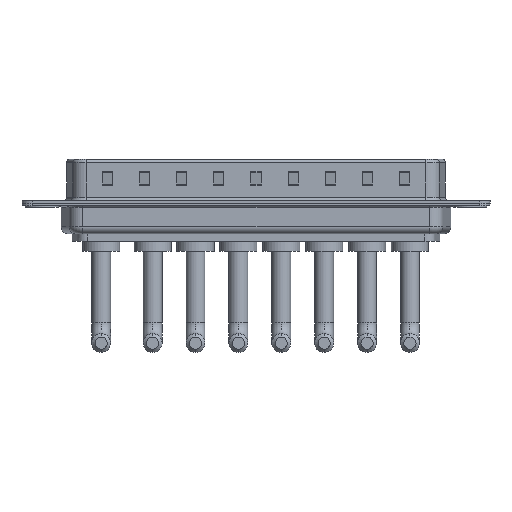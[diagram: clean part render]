
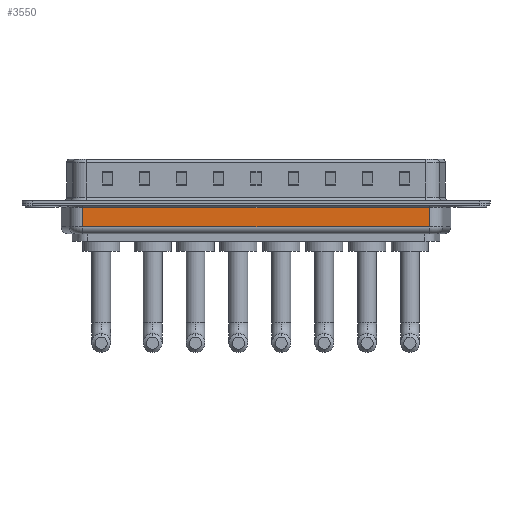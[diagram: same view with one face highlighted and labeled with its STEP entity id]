
A CAD part, front view. The second image highlights one B-rep face of the part: STEP entity #3550.
In plain terms, the highlighted planar face has unit normal (0, -1, 0).
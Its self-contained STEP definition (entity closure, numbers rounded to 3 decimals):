
#327 = ORIENTED_EDGE ( 'NONE', *, *, #14041, .T. ) ;
#1242 = CARTESIAN_POINT ( 'NONE',  ( 57.469, -5.35, -0.65 ) ) ;
#1476 = FACE_OUTER_BOUND ( 'NONE', #12144, .T. ) ;
#1701 = DIRECTION ( 'NONE',  ( 0., 0., 1. ) ) ;
#1750 = VERTEX_POINT ( 'NONE', #3593 ) ;
#2041 = EDGE_CURVE ( 'NONE', #8917, #1750, #11898, .T. ) ;
#2396 = VECTOR ( 'NONE', #1701, 1000. ) ;
#2888 = CARTESIAN_POINT ( 'NONE',  ( 57.469, -5.35, -4.5 ) ) ;
#3084 = AXIS2_PLACEMENT_3D ( 'NONE', #12461, #6816, #6740 ) ;
#3294 = DIRECTION ( 'NONE',  ( 1., 0., 0. ) ) ;
#3413 = CARTESIAN_POINT ( 'NONE',  ( 6.031, -5.35, -3.5 ) ) ;
#3550 = ADVANCED_FACE ( 'NONE', ( #1476 ), #6666, .F. ) ;
#3593 = CARTESIAN_POINT ( 'NONE',  ( 57.469, -5.35, -3.5 ) ) ;
#3693 = EDGE_CURVE ( 'NONE', #8917, #4304, #5151, .T. ) ;
#3713 = CARTESIAN_POINT ( 'NONE',  ( 6.031, -5.35, -4.5 ) ) ;
#3882 = ORIENTED_EDGE ( 'NONE', *, *, #3693, .F. ) ;
#4304 = VERTEX_POINT ( 'NONE', #13108 ) ;
#5053 = DIRECTION ( 'NONE',  ( 0., 0., 1. ) ) ;
#5151 = LINE ( 'NONE', #3713, #2396 ) ;
#6201 = LINE ( 'NONE', #2888, #11713 ) ;
#6666 = PLANE ( 'NONE',  #3084 ) ;
#6740 = DIRECTION ( 'NONE',  ( -1., 0., 0. ) ) ;
#6816 = DIRECTION ( 'NONE',  ( 0., 1., 0. ) ) ;
#8203 = ORIENTED_EDGE ( 'NONE', *, *, #2041, .T. ) ;
#8802 = VECTOR ( 'NONE', #3294, 1000. ) ;
#8917 = VERTEX_POINT ( 'NONE', #3413 ) ;
#8955 = ORIENTED_EDGE ( 'NONE', *, *, #12450, .T. ) ;
#9405 = DIRECTION ( 'NONE',  ( -1., 0., 0. ) ) ;
#10484 = CARTESIAN_POINT ( 'NONE',  ( 6.031, -5.35, -0.65 ) ) ;
#11342 = VERTEX_POINT ( 'NONE', #1242 ) ;
#11713 = VECTOR ( 'NONE', #5053, 1000. ) ;
#11726 = LINE ( 'NONE', #10484, #12117 ) ;
#11898 = LINE ( 'NONE', #13116, #8802 ) ;
#12117 = VECTOR ( 'NONE', #9405, 1000. ) ;
#12144 = EDGE_LOOP ( 'NONE', ( #3882, #8203, #327, #8955 ) ) ;
#12450 = EDGE_CURVE ( 'NONE', #11342, #4304, #11726, .T. ) ;
#12461 = CARTESIAN_POINT ( 'NONE',  ( 6.031, -5.35, -4.5 ) ) ;
#13108 = CARTESIAN_POINT ( 'NONE',  ( 6.031, -5.35, -0.65 ) ) ;
#13116 = CARTESIAN_POINT ( 'NONE',  ( 6.031, -5.35, -3.5 ) ) ;
#14041 = EDGE_CURVE ( 'NONE', #1750, #11342, #6201, .T. ) ;
